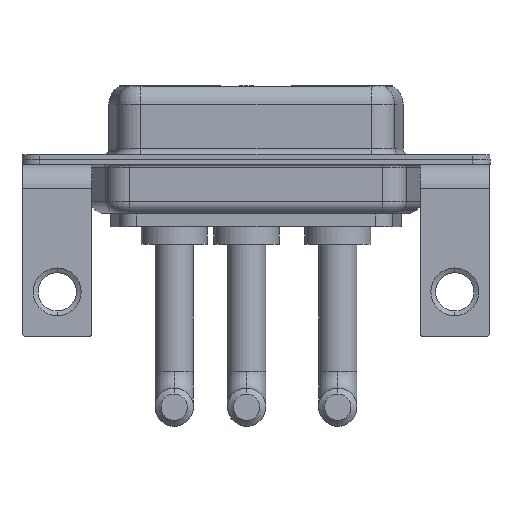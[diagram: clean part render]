
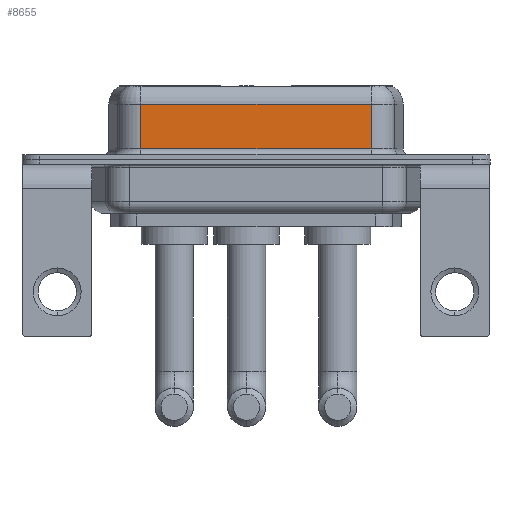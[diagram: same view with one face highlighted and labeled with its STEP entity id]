
A CAD part, front view. The second image highlights one B-rep face of the part: STEP entity #8655.
In plain terms, the highlighted planar face has unit normal (0, -1, 0).
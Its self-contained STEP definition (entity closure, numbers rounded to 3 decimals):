
#176 = LINE ( 'NONE', #12553, #7883 ) ;
#1506 = LINE ( 'NONE', #5995, #2075 ) ;
#2075 = VECTOR ( 'NONE', #11728, 1000. ) ;
#2791 = VERTEX_POINT ( 'NONE', #12044 ) ;
#3139 = VECTOR ( 'NONE', #3387, 1000. ) ;
#3316 = CARTESIAN_POINT ( 'NONE',  ( 26.287, -3.95, 4.65 ) ) ;
#3387 = DIRECTION ( 'NONE',  ( -1., 0., 0. ) ) ;
#3504 = CARTESIAN_POINT ( 'NONE',  ( 7.013, -3.95, 4.65 ) ) ;
#3593 = VECTOR ( 'NONE', #8739, 1000. ) ;
#3808 = FACE_OUTER_BOUND ( 'NONE', #9841, .T. ) ;
#3968 = ORIENTED_EDGE ( 'NONE', *, *, #5409, .T. ) ;
#4618 = ORIENTED_EDGE ( 'NONE', *, *, #9763, .T. ) ;
#4973 = DIRECTION ( 'NONE',  ( 0., 0., 1. ) ) ;
#5409 = EDGE_CURVE ( 'NONE', #13272, #10272, #8798, .T. ) ;
#5716 = CARTESIAN_POINT ( 'NONE',  ( 7.013, -3.95, 6.4 ) ) ;
#5822 = VERTEX_POINT ( 'NONE', #10036 ) ;
#5995 = CARTESIAN_POINT ( 'NONE',  ( 26.287, -3.95, 0.9 ) ) ;
#5997 = DIRECTION ( 'NONE',  ( 0., 0., -1. ) ) ;
#7033 = DIRECTION ( 'NONE',  ( 0., 1., 0. ) ) ;
#7274 = EDGE_CURVE ( 'NONE', #5822, #2791, #176, .T. ) ;
#7883 = VECTOR ( 'NONE', #5997, 1000. ) ;
#8080 = ORIENTED_EDGE ( 'NONE', *, *, #13432, .T. ) ;
#8285 = CARTESIAN_POINT ( 'NONE',  ( 26.287, -3.95, 6.4 ) ) ;
#8351 = PLANE ( 'NONE',  #10565 ) ;
#8655 = ADVANCED_FACE ( 'NONE', ( #3808 ), #8351, .F. ) ;
#8739 = DIRECTION ( 'NONE',  ( 0., 0., -1. ) ) ;
#8798 = LINE ( 'NONE', #5716, #3593 ) ;
#9763 = EDGE_CURVE ( 'NONE', #5822, #13272, #14567, .T. ) ;
#9841 = EDGE_LOOP ( 'NONE', ( #13871, #4618, #3968, #8080 ) ) ;
#10036 = CARTESIAN_POINT ( 'NONE',  ( 26.287, -3.95, 4.65 ) ) ;
#10272 = VERTEX_POINT ( 'NONE', #11588 ) ;
#10565 = AXIS2_PLACEMENT_3D ( 'NONE', #8285, #7033, #4973 ) ;
#11588 = CARTESIAN_POINT ( 'NONE',  ( 7.013, -3.95, 0.9 ) ) ;
#11728 = DIRECTION ( 'NONE',  ( 1., 0., 0. ) ) ;
#12044 = CARTESIAN_POINT ( 'NONE',  ( 26.287, -3.95, 0.9 ) ) ;
#12553 = CARTESIAN_POINT ( 'NONE',  ( 26.287, -3.95, 6.4 ) ) ;
#13272 = VERTEX_POINT ( 'NONE', #3504 ) ;
#13432 = EDGE_CURVE ( 'NONE', #10272, #2791, #1506, .T. ) ;
#13871 = ORIENTED_EDGE ( 'NONE', *, *, #7274, .F. ) ;
#14567 = LINE ( 'NONE', #3316, #3139 ) ;
